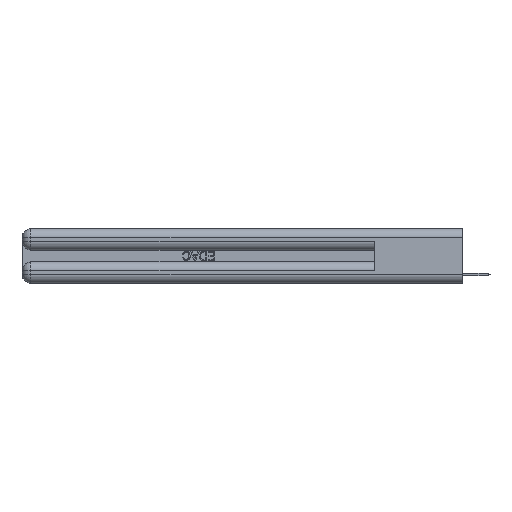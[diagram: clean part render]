
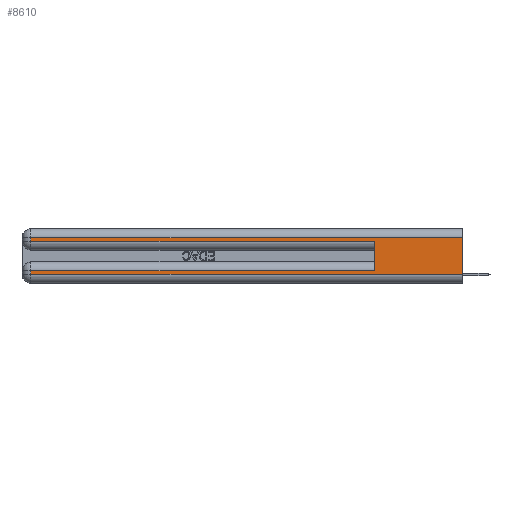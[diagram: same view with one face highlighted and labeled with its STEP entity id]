
A CAD part, left-side view. The second image highlights one B-rep face of the part: STEP entity #8610.
In plain terms, the highlighted planar face has unit normal (-1, 0, 0).
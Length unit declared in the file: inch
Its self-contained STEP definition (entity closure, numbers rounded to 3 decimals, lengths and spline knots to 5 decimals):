
#157 = VECTOR ( 'NONE', #27799, 39.37008 ) ;
#602 = VERTEX_POINT ( 'NONE', #16477 ) ;
#706 = EDGE_CURVE ( 'NONE', #2744, #2485, #29265, .T. ) ;
#983 = VECTOR ( 'NONE', #24733, 39.37008 ) ;
#986 = AXIS2_PLACEMENT_3D ( 'NONE', #16886, #5617, #23765 ) ;
#1504 = EDGE_CURVE ( 'NONE', #1854, #16624, #17672, .T. ) ;
#1854 = VERTEX_POINT ( 'NONE', #20279 ) ;
#2419 = EDGE_CURVE ( 'NONE', #19596, #2485, #10570, .T. ) ;
#2485 = VERTEX_POINT ( 'NONE', #16378 ) ;
#2744 = VERTEX_POINT ( 'NONE', #8497 ) ;
#3707 = DIRECTION ( 'NONE',  ( 0., 0., -1. ) ) ;
#5461 = VECTOR ( 'NONE', #19645, 39.37008 ) ;
#5617 = DIRECTION ( 'NONE',  ( 1., 0., 0. ) ) ;
#6382 = CARTESIAN_POINT ( 'NONE',  ( 0., 0.6, 0.145 ) ) ;
#6394 = ORIENTED_EDGE ( 'NONE', *, *, #706, .T. ) ;
#6883 = VECTOR ( 'NONE', #10296, 39.37008 ) ;
#7330 = EDGE_CURVE ( 'NONE', #19596, #17886, #22476, .T. ) ;
#7351 = ORIENTED_EDGE ( 'NONE', *, *, #23023, .T. ) ;
#7737 = ORIENTED_EDGE ( 'NONE', *, *, #11299, .T. ) ;
#7818 = PLANE ( 'NONE',  #986 ) ;
#8387 = VECTOR ( 'NONE', #22074, 39.37008 ) ;
#8497 = CARTESIAN_POINT ( 'NONE',  ( 0., 2.94, 0.06 ) ) ;
#8610 = ADVANCED_FACE ( 'NONE', ( #28218 ), #7818, .F. ) ;
#8890 = CARTESIAN_POINT ( 'NONE',  ( 0., 0., 0.06 ) ) ;
#10296 = DIRECTION ( 'NONE',  ( 0., 1., 0. ) ) ;
#10570 = LINE ( 'NONE', #24330, #8387 ) ;
#11299 = EDGE_CURVE ( 'NONE', #17886, #602, #23798, .T. ) ;
#11482 = CARTESIAN_POINT ( 'NONE',  ( 0., 2.94, 0.37 ) ) ;
#11821 = LINE ( 'NONE', #20979, #157 ) ;
#11835 = VECTOR ( 'NONE', #3707, 39.37008 ) ;
#12515 = CARTESIAN_POINT ( 'NONE',  ( 0., 0., 0.31 ) ) ;
#12740 = EDGE_LOOP ( 'NONE', ( #17058, #16971, #7737, #22492, #16066, #7351, #21729, #6394 ) ) ;
#13159 = EDGE_CURVE ( 'NONE', #23209, #2744, #25238, .T. ) ;
#13791 = CARTESIAN_POINT ( 'NONE',  ( 0., 0.6, 0.285 ) ) ;
#14142 = CARTESIAN_POINT ( 'NONE',  ( 0., 2.94, 0.085 ) ) ;
#14311 = LINE ( 'NONE', #21495, #6883 ) ;
#14406 = VECTOR ( 'NONE', #24970, 39.37008 ) ;
#15609 = CARTESIAN_POINT ( 'NONE',  ( 0., 0., 0.31 ) ) ;
#16066 = ORIENTED_EDGE ( 'NONE', *, *, #1504, .F. ) ;
#16378 = CARTESIAN_POINT ( 'NONE',  ( 0., 0., 0.06 ) ) ;
#16477 = CARTESIAN_POINT ( 'NONE',  ( 0., 2.94, 0.285 ) ) ;
#16624 = VERTEX_POINT ( 'NONE', #13791 ) ;
#16886 = CARTESIAN_POINT ( 'NONE',  ( 0., 0., 0.37 ) ) ;
#16971 = ORIENTED_EDGE ( 'NONE', *, *, #7330, .T. ) ;
#17058 = ORIENTED_EDGE ( 'NONE', *, *, #2419, .F. ) ;
#17212 = CARTESIAN_POINT ( 'NONE',  ( 0., 2.94, 0.37 ) ) ;
#17672 = LINE ( 'NONE', #6382, #5461 ) ;
#17886 = VERTEX_POINT ( 'NONE', #25145 ) ;
#19596 = VERTEX_POINT ( 'NONE', #12515 ) ;
#19645 = DIRECTION ( 'NONE',  ( 0., 0., 1. ) ) ;
#20279 = CARTESIAN_POINT ( 'NONE',  ( 0., 0.6, 0.085 ) ) ;
#20551 = EDGE_CURVE ( 'NONE', #602, #16624, #11821, .T. ) ;
#20979 = CARTESIAN_POINT ( 'NONE',  ( 0., 0., 0.285 ) ) ;
#21495 = CARTESIAN_POINT ( 'NONE',  ( 0., 0., 0.085 ) ) ;
#21729 = ORIENTED_EDGE ( 'NONE', *, *, #13159, .T. ) ;
#21842 = VECTOR ( 'NONE', #24805, 39.37008 ) ;
#22074 = DIRECTION ( 'NONE',  ( 0., 0., -1. ) ) ;
#22476 = LINE ( 'NONE', #15609, #983 ) ;
#22492 = ORIENTED_EDGE ( 'NONE', *, *, #20551, .T. ) ;
#23023 = EDGE_CURVE ( 'NONE', #1854, #23209, #14311, .T. ) ;
#23209 = VERTEX_POINT ( 'NONE', #14142 ) ;
#23765 = DIRECTION ( 'NONE',  ( 0., 0., -1. ) ) ;
#23798 = LINE ( 'NONE', #17212, #11835 ) ;
#24330 = CARTESIAN_POINT ( 'NONE',  ( 0., 0., 0.37 ) ) ;
#24733 = DIRECTION ( 'NONE',  ( 0., 1., 0. ) ) ;
#24805 = DIRECTION ( 'NONE',  ( 0., 0., -1. ) ) ;
#24970 = DIRECTION ( 'NONE',  ( 0., -1., 0. ) ) ;
#25145 = CARTESIAN_POINT ( 'NONE',  ( 0., 2.94, 0.31 ) ) ;
#25238 = LINE ( 'NONE', #11482, #21842 ) ;
#27799 = DIRECTION ( 'NONE',  ( 0., -1., 0. ) ) ;
#28218 = FACE_OUTER_BOUND ( 'NONE', #12740, .T. ) ;
#29265 = LINE ( 'NONE', #8890, #14406 ) ;
